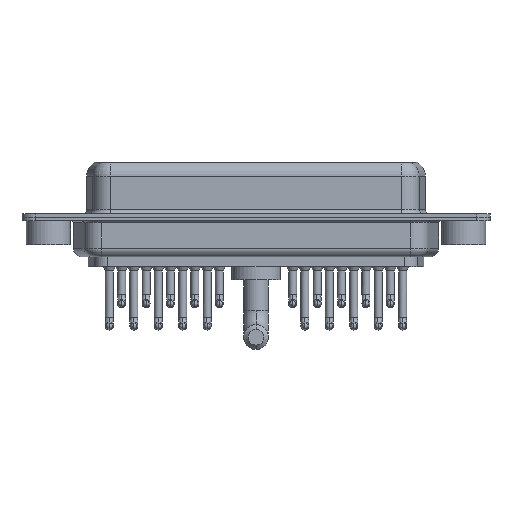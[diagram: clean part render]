
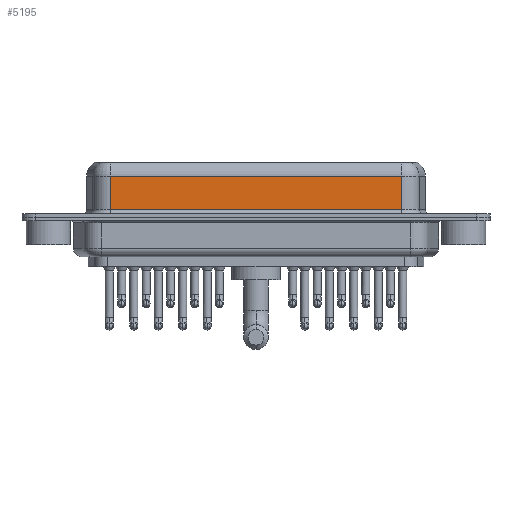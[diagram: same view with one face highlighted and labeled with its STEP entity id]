
A CAD part, front view. The second image highlights one B-rep face of the part: STEP entity #5195.
In plain terms, the highlighted planar face has unit normal (0, -1, 0).
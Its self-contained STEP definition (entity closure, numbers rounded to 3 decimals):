
#243 = AXIS2_PLACEMENT_3D ( 'NONE', #16838, #9864, #16950 ) ;
#583 = CARTESIAN_POINT ( 'NONE',  ( 40.037, -3.95, 6.4 ) ) ;
#951 = ORIENTED_EDGE ( 'NONE', *, *, #11169, .T. ) ;
#2800 = DIRECTION ( 'NONE',  ( 0., 0., -1. ) ) ;
#4384 = CARTESIAN_POINT ( 'NONE',  ( 40.037, -3.95, 0.9 ) ) ;
#4472 = PLANE ( 'NONE',  #243 ) ;
#4798 = EDGE_CURVE ( 'NONE', #5999, #11820, #14930, .T. ) ;
#4846 = CARTESIAN_POINT ( 'NONE',  ( 7.013, -3.95, 0.9 ) ) ;
#5195 = ADVANCED_FACE ( 'NONE', ( #11378 ), #4472, .F. ) ;
#5999 = VERTEX_POINT ( 'NONE', #4846 ) ;
#6337 = VERTEX_POINT ( 'NONE', #15937 ) ;
#7200 = CARTESIAN_POINT ( 'NONE',  ( 40.037, -3.95, 4.65 ) ) ;
#7951 = CARTESIAN_POINT ( 'NONE',  ( 7.013, -3.95, 6.4 ) ) ;
#8143 = VECTOR ( 'NONE', #9015, 1000. ) ;
#8813 = EDGE_LOOP ( 'NONE', ( #9856, #12433, #951, #17340 ) ) ;
#9015 = DIRECTION ( 'NONE',  ( -1., 0., 0. ) ) ;
#9856 = ORIENTED_EDGE ( 'NONE', *, *, #18977, .F. ) ;
#9864 = DIRECTION ( 'NONE',  ( 0., 1., 0. ) ) ;
#11169 = EDGE_CURVE ( 'NONE', #6337, #5999, #18601, .T. ) ;
#11378 = FACE_OUTER_BOUND ( 'NONE', #8813, .T. ) ;
#11407 = DIRECTION ( 'NONE',  ( 1., 0., 0. ) ) ;
#11532 = CARTESIAN_POINT ( 'NONE',  ( 40.037, -3.95, 4.65 ) ) ;
#11820 = VERTEX_POINT ( 'NONE', #16975 ) ;
#12421 = DIRECTION ( 'NONE',  ( 0., 0., -1. ) ) ;
#12433 = ORIENTED_EDGE ( 'NONE', *, *, #16702, .T. ) ;
#12695 = VECTOR ( 'NONE', #12421, 1000. ) ;
#14098 = LINE ( 'NONE', #7200, #8143 ) ;
#14930 = LINE ( 'NONE', #4384, #16580 ) ;
#15937 = CARTESIAN_POINT ( 'NONE',  ( 7.013, -3.95, 4.65 ) ) ;
#16498 = VECTOR ( 'NONE', #2800, 1000. ) ;
#16580 = VECTOR ( 'NONE', #11407, 1000. ) ;
#16702 = EDGE_CURVE ( 'NONE', #20680, #6337, #14098, .T. ) ;
#16838 = CARTESIAN_POINT ( 'NONE',  ( 40.037, -3.95, 6.4 ) ) ;
#16950 = DIRECTION ( 'NONE',  ( 0., 0., 1. ) ) ;
#16975 = CARTESIAN_POINT ( 'NONE',  ( 40.037, -3.95, 0.9 ) ) ;
#17340 = ORIENTED_EDGE ( 'NONE', *, *, #4798, .T. ) ;
#17783 = LINE ( 'NONE', #583, #12695 ) ;
#18601 = LINE ( 'NONE', #7951, #16498 ) ;
#18977 = EDGE_CURVE ( 'NONE', #20680, #11820, #17783, .T. ) ;
#20680 = VERTEX_POINT ( 'NONE', #11532 ) ;
